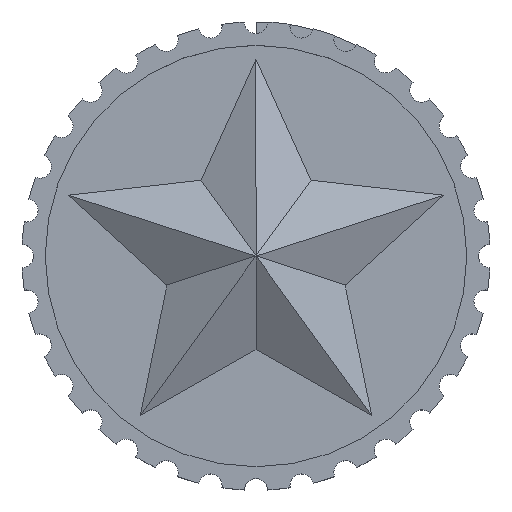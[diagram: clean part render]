
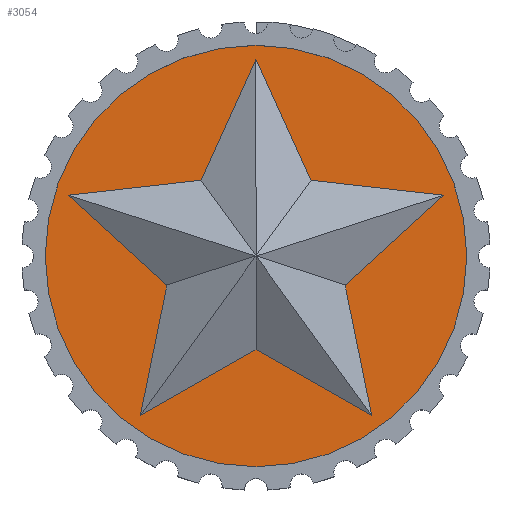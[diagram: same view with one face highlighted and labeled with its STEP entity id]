
A CAD part, top view. The second image highlights one B-rep face of the part: STEP entity #3054.
In plain terms, the highlighted planar face has unit normal (0, 0, 1).
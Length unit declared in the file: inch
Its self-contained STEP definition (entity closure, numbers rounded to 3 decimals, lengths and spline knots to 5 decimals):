
#14 = DIRECTION ( 'NONE',  ( -0.994, -0.112, 0. ) ) ;
#70 = VERTEX_POINT ( 'NONE', #2160 ) ;
#153 = EDGE_LOOP ( 'NONE', ( #1272, #2840, #2122, #3413, #686, #1942, #3516, #3598, #1541, #2247 ) ) ;
#163 = CARTESIAN_POINT ( 'NONE',  ( -0.30878, -0.425, 0.26063 ) ) ;
#230 = CARTESIAN_POINT ( 'NONE',  ( -0.5625, 0., 0.26063 ) ) ;
#322 = VECTOR ( 'NONE', #2162, 39.37008 ) ;
#362 = LINE ( 'NONE', #1724, #408 ) ;
#384 = LINE ( 'NONE', #2080, #3630 ) ;
#395 = CARTESIAN_POINT ( 'NONE',  ( 0.14695, 0.20225, 0.26063 ) ) ;
#408 = VECTOR ( 'NONE', #14, 39.37008 ) ;
#409 = DIRECTION ( 'NONE',  ( -0.414, -0.91, 0. ) ) ;
#425 = CARTESIAN_POINT ( 'NONE',  ( 0.30878, -0.425, 0.26063 ) ) ;
#443 = EDGE_CURVE ( 'NONE', #3683, #1496, #384, .T. ) ;
#488 = DIRECTION ( 'NONE',  ( 1., 0., 0. ) ) ;
#505 = EDGE_CURVE ( 'NONE', #536, #3155, #2774, .T. ) ;
#536 = VERTEX_POINT ( 'NONE', #230 ) ;
#567 = DIRECTION ( 'NONE',  ( 1., 0., 0. ) ) ;
#583 = DIRECTION ( 'NONE',  ( 0., 0., 1. ) ) ;
#615 = CARTESIAN_POINT ( 'NONE',  ( -0.49962, 0.16234, 0.26063 ) ) ;
#641 = AXIS2_PLACEMENT_3D ( 'NONE', #3162, #2052, #567 ) ;
#649 = EDGE_CURVE ( 'NONE', #672, #666, #1010, .T. ) ;
#666 = VERTEX_POINT ( 'NONE', #1826 ) ;
#672 = VERTEX_POINT ( 'NONE', #395 ) ;
#675 = LINE ( 'NONE', #1853, #3077 ) ;
#682 = CARTESIAN_POINT ( 'NONE',  ( 0.14695, 0.20225, 0.26063 ) ) ;
#686 = ORIENTED_EDGE ( 'NONE', *, *, #2698, .F. ) ;
#688 = EDGE_CURVE ( 'NONE', #3574, #3713, #1333, .T. ) ;
#851 = CIRCLE ( 'NONE', #1965, 0.5625 ) ;
#868 = DIRECTION ( 'NONE',  ( 1., 0., 0. ) ) ;
#936 = CARTESIAN_POINT ( 'NONE',  ( 0., -0.25, 0.26063 ) ) ;
#962 = DIRECTION ( 'NONE',  ( -0.414, 0.91, 0. ) ) ;
#983 = VECTOR ( 'NONE', #409, 39.37008 ) ;
#996 = LINE ( 'NONE', #1665, #322 ) ;
#1010 = LINE ( 'NONE', #682, #1608 ) ;
#1036 = AXIS2_PLACEMENT_3D ( 'NONE', #2788, #2780, #488 ) ;
#1048 = LINE ( 'NONE', #3680, #2807 ) ;
#1110 = VECTOR ( 'NONE', #2439, 39.37008 ) ;
#1224 = CARTESIAN_POINT ( 'NONE',  ( -0.14695, 0.20225, 0.26063 ) ) ;
#1233 = EDGE_CURVE ( 'NONE', #1496, #70, #675, .T. ) ;
#1244 = CARTESIAN_POINT ( 'NONE',  ( -0.30878, -0.425, 0.26063 ) ) ;
#1272 = ORIENTED_EDGE ( 'NONE', *, *, #2152, .F. ) ;
#1333 = LINE ( 'NONE', #2167, #2640 ) ;
#1493 = LINE ( 'NONE', #1244, #1110 ) ;
#1496 = VERTEX_POINT ( 'NONE', #1589 ) ;
#1541 = ORIENTED_EDGE ( 'NONE', *, *, #443, .F. ) ;
#1542 = EDGE_CURVE ( 'NONE', #3521, #3471, #362, .T. ) ;
#1589 = CARTESIAN_POINT ( 'NONE',  ( 0.23776, -0.07725, 0.26063 ) ) ;
#1608 = VECTOR ( 'NONE', #962, 39.37008 ) ;
#1665 = CARTESIAN_POINT ( 'NONE',  ( 0., -0.25, 0.26063 ) ) ;
#1705 = EDGE_CURVE ( 'NONE', #3155, #536, #851, .T. ) ;
#1724 = CARTESIAN_POINT ( 'NONE',  ( -0.14695, 0.20225, 0.26063 ) ) ;
#1753 = CARTESIAN_POINT ( 'NONE',  ( 0., 0., 0.26063 ) ) ;
#1826 = CARTESIAN_POINT ( 'NONE',  ( 0., 0.52533, 0.26063 ) ) ;
#1853 = CARTESIAN_POINT ( 'NONE',  ( 0.23776, -0.07725, 0.26063 ) ) ;
#1942 = ORIENTED_EDGE ( 'NONE', *, *, #649, .F. ) ;
#1965 = AXIS2_PLACEMENT_3D ( 'NONE', #1753, #583, #868 ) ;
#2022 = CARTESIAN_POINT ( 'NONE',  ( 0.5625, 0., 0.26063 ) ) ;
#2031 = EDGE_LOOP ( 'NONE', ( #2932, #2376 ) ) ;
#2042 = LINE ( 'NONE', #3621, #2899 ) ;
#2052 = DIRECTION ( 'NONE',  ( 0., 0., 1. ) ) ;
#2080 = CARTESIAN_POINT ( 'NONE',  ( 0.30878, -0.425, 0.26063 ) ) ;
#2122 = ORIENTED_EDGE ( 'NONE', *, *, #2891, .F. ) ;
#2152 = EDGE_CURVE ( 'NONE', #3713, #2161, #1493, .T. ) ;
#2160 = CARTESIAN_POINT ( 'NONE',  ( 0.49962, 0.16234, 0.26063 ) ) ;
#2161 = VERTEX_POINT ( 'NONE', #936 ) ;
#2162 = DIRECTION ( 'NONE',  ( 0.87, -0.493, 0. ) ) ;
#2167 = CARTESIAN_POINT ( 'NONE',  ( -0.23776, -0.07725, 0.26063 ) ) ;
#2247 = ORIENTED_EDGE ( 'NONE', *, *, #3719, .F. ) ;
#2360 = FACE_BOUND ( 'NONE', #153, .T. ) ;
#2376 = ORIENTED_EDGE ( 'NONE', *, *, #505, .T. ) ;
#2439 = DIRECTION ( 'NONE',  ( 0.87, 0.493, 0. ) ) ;
#2525 = LINE ( 'NONE', #3591, #983 ) ;
#2640 = VECTOR ( 'NONE', #2726, 39.37008 ) ;
#2698 = EDGE_CURVE ( 'NONE', #666, #3521, #2525, .T. ) ;
#2726 = DIRECTION ( 'NONE',  ( -0.2, -0.98, 0. ) ) ;
#2774 = CIRCLE ( 'NONE', #1036, 0.5625 ) ;
#2780 = DIRECTION ( 'NONE',  ( 0., 0., 1. ) ) ;
#2788 = CARTESIAN_POINT ( 'NONE',  ( 0., 0., 0.26063 ) ) ;
#2791 = EDGE_CURVE ( 'NONE', #70, #672, #2042, .T. ) ;
#2807 = VECTOR ( 'NONE', #3693, 39.37008 ) ;
#2840 = ORIENTED_EDGE ( 'NONE', *, *, #688, .F. ) ;
#2891 = EDGE_CURVE ( 'NONE', #3471, #3574, #1048, .T. ) ;
#2899 = VECTOR ( 'NONE', #3051, 39.37008 ) ;
#2932 = ORIENTED_EDGE ( 'NONE', *, *, #1705, .T. ) ;
#2988 = DIRECTION ( 'NONE',  ( -0.2, 0.98, 0. ) ) ;
#3051 = DIRECTION ( 'NONE',  ( -0.994, 0.112, 0. ) ) ;
#3054 = ADVANCED_FACE ( 'NONE', ( #3695, #2360 ), #3175, .T. ) ;
#3077 = VECTOR ( 'NONE', #3277, 39.37008 ) ;
#3155 = VERTEX_POINT ( 'NONE', #2022 ) ;
#3162 = CARTESIAN_POINT ( 'NONE',  ( 0., 0., 0.26063 ) ) ;
#3175 = PLANE ( 'NONE',  #641 ) ;
#3277 = DIRECTION ( 'NONE',  ( 0.738, 0.675, 0. ) ) ;
#3413 = ORIENTED_EDGE ( 'NONE', *, *, #1542, .F. ) ;
#3471 = VERTEX_POINT ( 'NONE', #615 ) ;
#3516 = ORIENTED_EDGE ( 'NONE', *, *, #2791, .F. ) ;
#3521 = VERTEX_POINT ( 'NONE', #1224 ) ;
#3531 = CARTESIAN_POINT ( 'NONE',  ( -0.23776, -0.07725, 0.26063 ) ) ;
#3574 = VERTEX_POINT ( 'NONE', #3531 ) ;
#3591 = CARTESIAN_POINT ( 'NONE',  ( 0., 0.52533, 0.26063 ) ) ;
#3598 = ORIENTED_EDGE ( 'NONE', *, *, #1233, .F. ) ;
#3621 = CARTESIAN_POINT ( 'NONE',  ( 0.49962, 0.16234, 0.26063 ) ) ;
#3630 = VECTOR ( 'NONE', #2988, 39.37008 ) ;
#3680 = CARTESIAN_POINT ( 'NONE',  ( -0.49962, 0.16234, 0.26063 ) ) ;
#3683 = VERTEX_POINT ( 'NONE', #425 ) ;
#3693 = DIRECTION ( 'NONE',  ( 0.738, -0.675, 0. ) ) ;
#3695 = FACE_OUTER_BOUND ( 'NONE', #2031, .T. ) ;
#3713 = VERTEX_POINT ( 'NONE', #163 ) ;
#3719 = EDGE_CURVE ( 'NONE', #2161, #3683, #996, .T. ) ;
